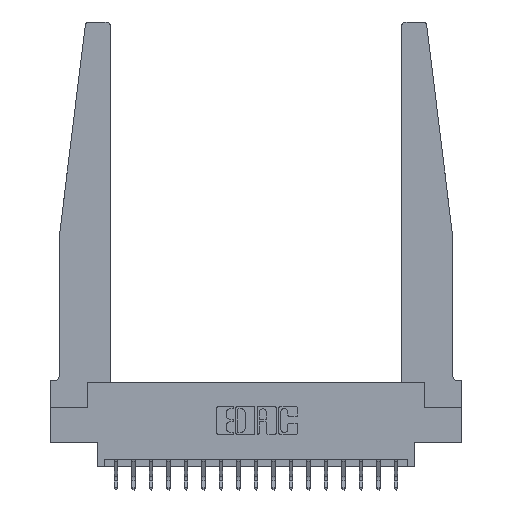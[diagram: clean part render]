
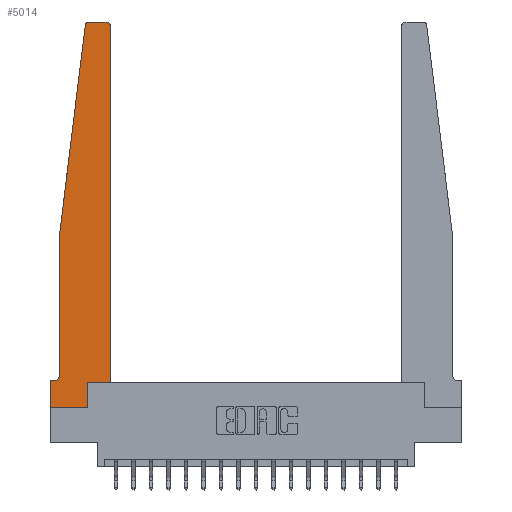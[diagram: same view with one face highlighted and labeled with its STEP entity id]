
A CAD part, top view. The second image highlights one B-rep face of the part: STEP entity #5014.
In plain terms, the highlighted planar face has unit normal (0, 0, 1).
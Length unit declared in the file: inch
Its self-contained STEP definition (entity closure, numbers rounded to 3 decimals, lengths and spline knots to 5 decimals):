
#137 = CARTESIAN_POINT ( 'NONE',  ( 0.27653, 2.75, 0.37 ) ) ;
#454 = VERTEX_POINT ( 'NONE', #16487 ) ;
#745 = EDGE_CURVE ( 'NONE', #759, #9762, #15042, .T. ) ;
#759 = VERTEX_POINT ( 'NONE', #8883 ) ;
#987 = AXIS2_PLACEMENT_3D ( 'NONE', #1976, #9698, #6338 ) ;
#1164 = EDGE_CURVE ( 'NONE', #454, #12290, #13009, .T. ) ;
#1196 = DIRECTION ( 'NONE',  ( 1., 0., 0. ) ) ;
#1239 = DIRECTION ( 'NONE',  ( 0., 1., 0. ) ) ;
#1419 = EDGE_CURVE ( 'NONE', #1988, #4413, #11266, .T. ) ;
#1513 = ORIENTED_EDGE ( 'NONE', *, *, #1419, .T. ) ;
#1976 = CARTESIAN_POINT ( 'NONE',  ( 0.27653, 2.72, 0.37 ) ) ;
#1988 = VERTEX_POINT ( 'NONE', #4754 ) ;
#2023 = LINE ( 'NONE', #3747, #8911 ) ;
#2066 = DIRECTION ( 'NONE',  ( 1., 0., 0. ) ) ;
#2123 = VECTOR ( 'NONE', #4382, 39.37008 ) ;
#2342 = CIRCLE ( 'NONE', #17536, 0.03 ) ;
#2854 = LINE ( 'NONE', #9247, #2123 ) ;
#2864 = CARTESIAN_POINT ( 'NONE',  ( 0.2605, 0.18, 0.37 ) ) ;
#3254 = DIRECTION ( 'NONE',  ( -1., 0., 0. ) ) ;
#3404 = ORIENTED_EDGE ( 'NONE', *, *, #19581, .T. ) ;
#3603 = EDGE_CURVE ( 'NONE', #17799, #5461, #5251, .T. ) ;
#3608 = EDGE_LOOP ( 'NONE', ( #1513, #8974, #8293, #3404, #17709, #5558, #12206, #9693, #18579, #3702, #10543, #7159 ) ) ;
#3683 = VECTOR ( 'NONE', #11091, 39.37008 ) ;
#3702 = ORIENTED_EDGE ( 'NONE', *, *, #1164, .T. ) ;
#3747 = CARTESIAN_POINT ( 'NONE',  ( 0., 0., 0.37 ) ) ;
#3885 = VECTOR ( 'NONE', #10355, 39.37008 ) ;
#4092 = CARTESIAN_POINT ( 'NONE',  ( 0.2605, 0., 0.37 ) ) ;
#4382 = DIRECTION ( 'NONE',  ( 0., -1., 0. ) ) ;
#4413 = VERTEX_POINT ( 'NONE', #137 ) ;
#4754 = CARTESIAN_POINT ( 'NONE',  ( 0.395, 2.75, 0.37 ) ) ;
#4828 = EDGE_CURVE ( 'NONE', #16466, #454, #6101, .T. ) ;
#4832 = CARTESIAN_POINT ( 'NONE',  ( 0.425, 0.18, 0.37 ) ) ;
#5014 = ADVANCED_FACE ( 'NONE', ( #6789 ), #5762, .T. ) ;
#5251 = LINE ( 'NONE', #13145, #15068 ) ;
#5461 = VERTEX_POINT ( 'NONE', #12018 ) ;
#5558 = ORIENTED_EDGE ( 'NONE', *, *, #8929, .T. ) ;
#5762 = PLANE ( 'NONE',  #17475 ) ;
#6101 = LINE ( 'NONE', #2864, #10456 ) ;
#6136 = CARTESIAN_POINT ( 'NONE',  ( 0.24675, 2.72367, 0.37 ) ) ;
#6338 = DIRECTION ( 'NONE',  ( 1., 0., 0. ) ) ;
#6402 = CARTESIAN_POINT ( 'NONE',  ( 0.015, 0.1875, 0.37 ) ) ;
#6536 = DIRECTION ( 'NONE',  ( 0., 0., 1. ) ) ;
#6656 = DIRECTION ( 'NONE',  ( -1., 0., 0. ) ) ;
#6709 = CARTESIAN_POINT ( 'NONE',  ( 0.25, 2.75, 0.37 ) ) ;
#6789 = FACE_OUTER_BOUND ( 'NONE', #3608, .T. ) ;
#6928 = VERTEX_POINT ( 'NONE', #6136 ) ;
#7159 = ORIENTED_EDGE ( 'NONE', *, *, #13467, .T. ) ;
#7536 = CARTESIAN_POINT ( 'NONE',  ( 0., 0.1875, 0.37 ) ) ;
#8175 = CARTESIAN_POINT ( 'NONE',  ( 0.015, 0.2375, 0.37 ) ) ;
#8293 = ORIENTED_EDGE ( 'NONE', *, *, #12473, .T. ) ;
#8721 = DIRECTION ( 'NONE',  ( 0., 0., 1. ) ) ;
#8736 = VERTEX_POINT ( 'NONE', #19983 ) ;
#8883 = CARTESIAN_POINT ( 'NONE',  ( 0.065, 0.2375, 0.37 ) ) ;
#8911 = VECTOR ( 'NONE', #18943, 39.37008 ) ;
#8929 = EDGE_CURVE ( 'NONE', #9762, #17799, #14807, .T. ) ;
#8974 = ORIENTED_EDGE ( 'NONE', *, *, #11087, .T. ) ;
#9247 = CARTESIAN_POINT ( 'NONE',  ( 0.065, 1.25, 0.37 ) ) ;
#9321 = CARTESIAN_POINT ( 'NONE',  ( 0.065, 1.25, 0.37 ) ) ;
#9693 = ORIENTED_EDGE ( 'NONE', *, *, #16704, .T. ) ;
#9698 = DIRECTION ( 'NONE',  ( 0., 0., 1. ) ) ;
#9762 = VERTEX_POINT ( 'NONE', #6402 ) ;
#10199 = AXIS2_PLACEMENT_3D ( 'NONE', #8175, #14340, #6656 ) ;
#10355 = DIRECTION ( 'NONE',  ( -1., 0., 0. ) ) ;
#10456 = VECTOR ( 'NONE', #1239, 39.37008 ) ;
#10543 = ORIENTED_EDGE ( 'NONE', *, *, #19936, .T. ) ;
#11087 = EDGE_CURVE ( 'NONE', #4413, #6928, #14584, .T. ) ;
#11091 = DIRECTION ( 'NONE',  ( 1., 0., 0. ) ) ;
#11266 = LINE ( 'NONE', #6709, #16043 ) ;
#11427 = DIRECTION ( 'NONE',  ( 0., -1., 0. ) ) ;
#11858 = VECTOR ( 'NONE', #20008, 39.37008 ) ;
#12018 = CARTESIAN_POINT ( 'NONE',  ( 0., 0., 0.37 ) ) ;
#12145 = CARTESIAN_POINT ( 'NONE',  ( 0., 0.1875, 0.37 ) ) ;
#12206 = ORIENTED_EDGE ( 'NONE', *, *, #3603, .T. ) ;
#12290 = VERTEX_POINT ( 'NONE', #16610 ) ;
#12473 = EDGE_CURVE ( 'NONE', #6928, #16805, #13867, .T. ) ;
#13009 = LINE ( 'NONE', #19187, #3683 ) ;
#13145 = CARTESIAN_POINT ( 'NONE',  ( 0., 0., 0.37 ) ) ;
#13467 = EDGE_CURVE ( 'NONE', #8736, #1988, #2342, .T. ) ;
#13867 = LINE ( 'NONE', #9321, #15574 ) ;
#14047 = LINE ( 'NONE', #4832, #11858 ) ;
#14340 = DIRECTION ( 'NONE',  ( 0., 0., -1. ) ) ;
#14584 = CIRCLE ( 'NONE', #987, 0.03 ) ;
#14807 = LINE ( 'NONE', #16322, #3885 ) ;
#15042 = CIRCLE ( 'NONE', #10199, 0.05 ) ;
#15068 = VECTOR ( 'NONE', #11427, 39.37008 ) ;
#15492 = DIRECTION ( 'NONE',  ( -0.122, -0.992, 0. ) ) ;
#15574 = VECTOR ( 'NONE', #15492, 39.37008 ) ;
#16043 = VECTOR ( 'NONE', #3254, 39.37008 ) ;
#16322 = CARTESIAN_POINT ( 'NONE',  ( 0.065, 0.1875, 0.37 ) ) ;
#16466 = VERTEX_POINT ( 'NONE', #4092 ) ;
#16487 = CARTESIAN_POINT ( 'NONE',  ( 0.2605, 0.18, 0.37 ) ) ;
#16610 = CARTESIAN_POINT ( 'NONE',  ( 0.425, 0.18, 0.37 ) ) ;
#16704 = EDGE_CURVE ( 'NONE', #5461, #16466, #2023, .T. ) ;
#16805 = VERTEX_POINT ( 'NONE', #18230 ) ;
#17362 = CARTESIAN_POINT ( 'NONE',  ( 0.395, 2.72, 0.37 ) ) ;
#17475 = AXIS2_PLACEMENT_3D ( 'NONE', #12145, #8721, #1196 ) ;
#17536 = AXIS2_PLACEMENT_3D ( 'NONE', #17362, #6536, #2066 ) ;
#17709 = ORIENTED_EDGE ( 'NONE', *, *, #745, .T. ) ;
#17799 = VERTEX_POINT ( 'NONE', #7536 ) ;
#18230 = CARTESIAN_POINT ( 'NONE',  ( 0.065, 1.25, 0.37 ) ) ;
#18579 = ORIENTED_EDGE ( 'NONE', *, *, #4828, .T. ) ;
#18943 = DIRECTION ( 'NONE',  ( 1., 0., 0. ) ) ;
#19187 = CARTESIAN_POINT ( 'NONE',  ( 0.425, 0.18, 0.37 ) ) ;
#19581 = EDGE_CURVE ( 'NONE', #16805, #759, #2854, .T. ) ;
#19936 = EDGE_CURVE ( 'NONE', #12290, #8736, #14047, .T. ) ;
#19983 = CARTESIAN_POINT ( 'NONE',  ( 0.425, 2.72, 0.37 ) ) ;
#20008 = DIRECTION ( 'NONE',  ( 0., 1., 0. ) ) ;
